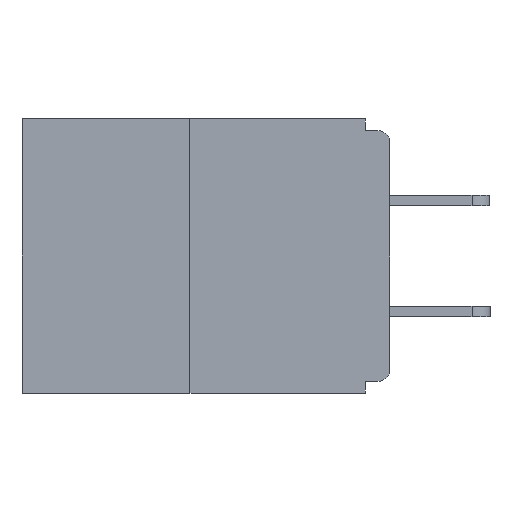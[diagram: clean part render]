
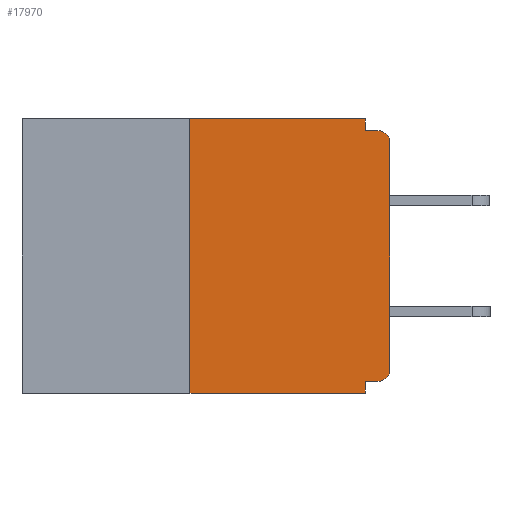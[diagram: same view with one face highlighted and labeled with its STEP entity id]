
A CAD part, left-side view. The second image highlights one B-rep face of the part: STEP entity #17970.
In plain terms, the highlighted planar face has unit normal (-1, 0, 0).
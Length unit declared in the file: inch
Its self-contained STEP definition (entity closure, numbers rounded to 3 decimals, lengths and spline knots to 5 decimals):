
#300 = ORIENTED_EDGE ( 'NONE', *, *, #24201, .F. ) ;
#731 = EDGE_CURVE ( 'NONE', #11676, #11222, #20572, .T. ) ;
#1365 = CARTESIAN_POINT ( 'NONE',  ( 0., 0.031, 0. ) ) ;
#1520 = LINE ( 'NONE', #12087, #16601 ) ;
#1745 = DIRECTION ( 'NONE',  ( 0., 1., 0. ) ) ;
#2015 = DIRECTION ( 'NONE',  ( 0., 0., 1. ) ) ;
#2054 = LINE ( 'NONE', #13261, #21544 ) ;
#2305 = ORIENTED_EDGE ( 'NONE', *, *, #6299, .T. ) ;
#2672 = VERTEX_POINT ( 'NONE', #23665 ) ;
#3093 = EDGE_CURVE ( 'NONE', #11222, #14345, #1520, .T. ) ;
#3451 = AXIS2_PLACEMENT_3D ( 'NONE', #9618, #24311, #14987 ) ;
#3606 = LINE ( 'NONE', #23772, #12098 ) ;
#3923 = DIRECTION ( 'NONE',  ( -1., 0., 0. ) ) ;
#4126 = CARTESIAN_POINT ( 'NONE',  ( 0., 0., -0.015 ) ) ;
#4769 = LINE ( 'NONE', #12926, #6270 ) ;
#5569 = CARTESIAN_POINT ( 'NONE',  ( 0., 0.031, -0.343 ) ) ;
#5731 = CARTESIAN_POINT ( 'NONE',  ( 0., 0.031, -0.015 ) ) ;
#5849 = AXIS2_PLACEMENT_3D ( 'NONE', #19979, #16417, #7001 ) ;
#6270 = VECTOR ( 'NONE', #1745, 39.37008 ) ;
#6299 = EDGE_CURVE ( 'NONE', #2672, #13695, #3606, .T. ) ;
#6595 = DIRECTION ( 'NONE',  ( 0., 0., -1. ) ) ;
#6879 = FACE_OUTER_BOUND ( 'NONE', #11103, .T. ) ;
#7001 = DIRECTION ( 'NONE',  ( 0., 0., -1. ) ) ;
#7025 = ORIENTED_EDGE ( 'NONE', *, *, #7573, .F. ) ;
#7573 = EDGE_CURVE ( 'NONE', #11430, #13695, #23015, .T. ) ;
#7589 = CARTESIAN_POINT ( 'NONE',  ( 0., 0.031, -0.328 ) ) ;
#7688 = CARTESIAN_POINT ( 'NONE',  ( 0., 0.015, -0.328 ) ) ;
#7970 = CARTESIAN_POINT ( 'NONE',  ( 0., 0.25, 0. ) ) ;
#8523 = ORIENTED_EDGE ( 'NONE', *, *, #3093, .F. ) ;
#9107 = VERTEX_POINT ( 'NONE', #23887 ) ;
#9532 = ORIENTED_EDGE ( 'NONE', *, *, #16964, .T. ) ;
#9618 = CARTESIAN_POINT ( 'NONE',  ( 0., 0.015, -0.03 ) ) ;
#9937 = VECTOR ( 'NONE', #14202, 39.37008 ) ;
#9992 = VECTOR ( 'NONE', #22981, 39.37008 ) ;
#10606 = PLANE ( 'NONE',  #5849 ) ;
#10819 = EDGE_CURVE ( 'NONE', #15706, #15080, #2054, .T. ) ;
#10879 = LINE ( 'NONE', #4126, #13934 ) ;
#11083 = ORIENTED_EDGE ( 'NONE', *, *, #18171, .T. ) ;
#11103 = EDGE_LOOP ( 'NONE', ( #21245, #300, #2305, #7025, #20352, #11083, #24232, #9532, #17647, #8523 ) ) ;
#11222 = VERTEX_POINT ( 'NONE', #1365 ) ;
#11430 = VERTEX_POINT ( 'NONE', #7589 ) ;
#11676 = VERTEX_POINT ( 'NONE', #21546 ) ;
#12087 = CARTESIAN_POINT ( 'NONE',  ( 0., 0.031, 0. ) ) ;
#12098 = VECTOR ( 'NONE', #23929, 39.37008 ) ;
#12414 = AXIS2_PLACEMENT_3D ( 'NONE', #13255, #3923, #21153 ) ;
#12584 = CARTESIAN_POINT ( 'NONE',  ( 0., 0.031, -0.343 ) ) ;
#12926 = CARTESIAN_POINT ( 'NONE',  ( 0., 0., -0.328 ) ) ;
#13255 = CARTESIAN_POINT ( 'NONE',  ( 0., 0.015, -0.313 ) ) ;
#13261 = CARTESIAN_POINT ( 'NONE',  ( 0., 0., 0. ) ) ;
#13300 = DIRECTION ( 'NONE',  ( 0., -1., 0. ) ) ;
#13695 = VERTEX_POINT ( 'NONE', #5569 ) ;
#13828 = CARTESIAN_POINT ( 'NONE',  ( 0., 0., -0.313 ) ) ;
#13829 = CARTESIAN_POINT ( 'NONE',  ( 0., 0., -0.03 ) ) ;
#13934 = VECTOR ( 'NONE', #13300, 39.37008 ) ;
#14202 = DIRECTION ( 'NONE',  ( 0., -1., 0. ) ) ;
#14345 = VERTEX_POINT ( 'NONE', #5731 ) ;
#14382 = EDGE_CURVE ( 'NONE', #22337, #11430, #4769, .T. ) ;
#14913 = CIRCLE ( 'NONE', #3451, 0.015 ) ;
#14987 = DIRECTION ( 'NONE',  ( 0., 0., -1. ) ) ;
#15080 = VERTEX_POINT ( 'NONE', #13829 ) ;
#15706 = VERTEX_POINT ( 'NONE', #13828 ) ;
#16041 = DIRECTION ( 'NONE',  ( 0., 0., -1. ) ) ;
#16417 = DIRECTION ( 'NONE',  ( 1., 0., 0. ) ) ;
#16601 = VECTOR ( 'NONE', #6595, 39.37008 ) ;
#16964 = EDGE_CURVE ( 'NONE', #15080, #9107, #14913, .T. ) ;
#17647 = ORIENTED_EDGE ( 'NONE', *, *, #23381, .F. ) ;
#17966 = VECTOR ( 'NONE', #16041, 39.37008 ) ;
#17970 = ADVANCED_FACE ( 'NONE', ( #6879 ), #10606, .F. ) ;
#18171 = EDGE_CURVE ( 'NONE', #22337, #15706, #22547, .T. ) ;
#19979 = CARTESIAN_POINT ( 'NONE',  ( 0., 0.46, 0. ) ) ;
#20027 = LINE ( 'NONE', #7970, #9992 ) ;
#20352 = ORIENTED_EDGE ( 'NONE', *, *, #14382, .F. ) ;
#20572 = LINE ( 'NONE', #23485, #9937 ) ;
#21153 = DIRECTION ( 'NONE',  ( 0., 0., -1. ) ) ;
#21245 = ORIENTED_EDGE ( 'NONE', *, *, #731, .F. ) ;
#21544 = VECTOR ( 'NONE', #2015, 39.37008 ) ;
#21546 = CARTESIAN_POINT ( 'NONE',  ( 0., 0.25, 0. ) ) ;
#22337 = VERTEX_POINT ( 'NONE', #7688 ) ;
#22547 = CIRCLE ( 'NONE', #12414, 0.015 ) ;
#22981 = DIRECTION ( 'NONE',  ( 0., 0., 1. ) ) ;
#23015 = LINE ( 'NONE', #12584, #17966 ) ;
#23381 = EDGE_CURVE ( 'NONE', #14345, #9107, #10879, .T. ) ;
#23485 = CARTESIAN_POINT ( 'NONE',  ( 0., 0.46, 0. ) ) ;
#23665 = CARTESIAN_POINT ( 'NONE',  ( 0., 0.25, -0.343 ) ) ;
#23772 = CARTESIAN_POINT ( 'NONE',  ( 0., 0.46, -0.343 ) ) ;
#23887 = CARTESIAN_POINT ( 'NONE',  ( 0., 0.015, -0.015 ) ) ;
#23929 = DIRECTION ( 'NONE',  ( 0., -1., 0. ) ) ;
#24201 = EDGE_CURVE ( 'NONE', #2672, #11676, #20027, .T. ) ;
#24232 = ORIENTED_EDGE ( 'NONE', *, *, #10819, .T. ) ;
#24311 = DIRECTION ( 'NONE',  ( -1., 0., 0. ) ) ;
